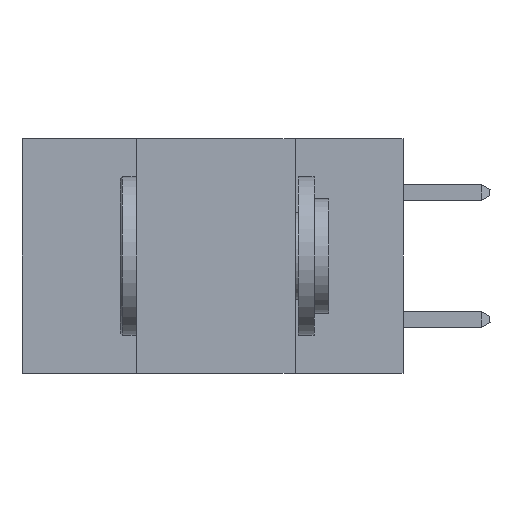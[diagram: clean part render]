
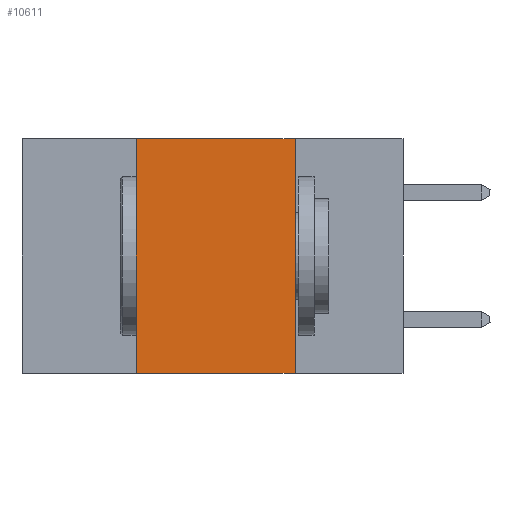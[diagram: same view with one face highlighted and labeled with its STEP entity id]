
A CAD part, left-side view. The second image highlights one B-rep face of the part: STEP entity #10611.
In plain terms, the highlighted planar face has unit normal (-1, 0, 0).
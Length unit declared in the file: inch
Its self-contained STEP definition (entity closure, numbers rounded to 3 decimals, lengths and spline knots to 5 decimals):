
#598 = LINE ( 'NONE', #3496, #10407 ) ;
#1371 = ORIENTED_EDGE ( 'NONE', *, *, #10993, .F. ) ;
#2293 = CARTESIAN_POINT ( 'NONE',  ( 0., 0.17, 0. ) ) ;
#2366 = DIRECTION ( 'NONE',  ( 0., 0., -1. ) ) ;
#2465 = ORIENTED_EDGE ( 'NONE', *, *, #4563, .F. ) ;
#2823 = EDGE_CURVE ( 'NONE', #6773, #3321, #598, .T. ) ;
#2916 = DIRECTION ( 'NONE',  ( 0., 0., -1. ) ) ;
#3248 = DIRECTION ( 'NONE',  ( 1., 0., 0. ) ) ;
#3321 = VERTEX_POINT ( 'NONE', #6888 ) ;
#3407 = ORIENTED_EDGE ( 'NONE', *, *, #11151, .T. ) ;
#3429 = VERTEX_POINT ( 'NONE', #11251 ) ;
#3496 = CARTESIAN_POINT ( 'NONE',  ( 0., 0.42, 0. ) ) ;
#3832 = ORIENTED_EDGE ( 'NONE', *, *, #2823, .F. ) ;
#4097 = VECTOR ( 'NONE', #4117, 39.37008 ) ;
#4117 = DIRECTION ( 'NONE',  ( 0., -1., 0. ) ) ;
#4296 = VERTEX_POINT ( 'NONE', #2293 ) ;
#4504 = DIRECTION ( 'NONE',  ( 0., 0., 1. ) ) ;
#4563 = EDGE_CURVE ( 'NONE', #3321, #4296, #7134, .T. ) ;
#5777 = CARTESIAN_POINT ( 'NONE',  ( 0., 0.42, -0.37 ) ) ;
#5805 = VECTOR ( 'NONE', #12099, 39.37008 ) ;
#5836 = CARTESIAN_POINT ( 'NONE',  ( 0., 0.17, 0. ) ) ;
#6305 = LINE ( 'NONE', #11677, #4097 ) ;
#6773 = VERTEX_POINT ( 'NONE', #5777 ) ;
#6888 = CARTESIAN_POINT ( 'NONE',  ( 0., 0.42, 0. ) ) ;
#7125 = PLANE ( 'NONE',  #7971 ) ;
#7134 = LINE ( 'NONE', #12057, #5805 ) ;
#7787 = FACE_OUTER_BOUND ( 'NONE', #11817, .T. ) ;
#7971 = AXIS2_PLACEMENT_3D ( 'NONE', #9880, #3248, #2366 ) ;
#8990 = VECTOR ( 'NONE', #2916, 39.37008 ) ;
#9880 = CARTESIAN_POINT ( 'NONE',  ( 0., 0.6, 0. ) ) ;
#10407 = VECTOR ( 'NONE', #4504, 39.37008 ) ;
#10611 = ADVANCED_FACE ( 'NONE', ( #7787 ), #7125, .F. ) ;
#10993 = EDGE_CURVE ( 'NONE', #4296, #3429, #12130, .T. ) ;
#11151 = EDGE_CURVE ( 'NONE', #6773, #3429, #6305, .T. ) ;
#11251 = CARTESIAN_POINT ( 'NONE',  ( 0., 0.17, -0.37 ) ) ;
#11677 = CARTESIAN_POINT ( 'NONE',  ( 0., 0.6, -0.37 ) ) ;
#11817 = EDGE_LOOP ( 'NONE', ( #1371, #2465, #3832, #3407 ) ) ;
#12057 = CARTESIAN_POINT ( 'NONE',  ( 0., 0.6, 0. ) ) ;
#12099 = DIRECTION ( 'NONE',  ( 0., -1., 0. ) ) ;
#12130 = LINE ( 'NONE', #5836, #8990 ) ;
